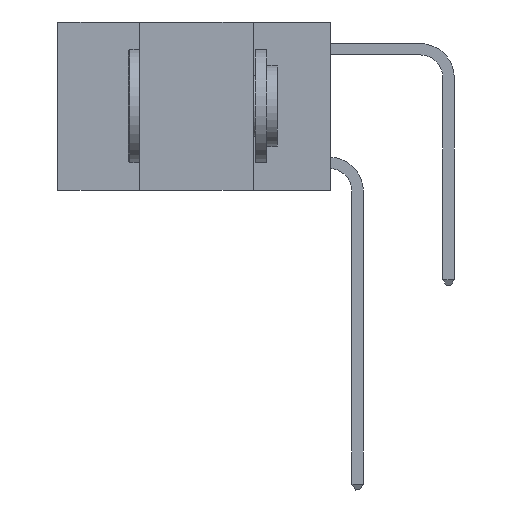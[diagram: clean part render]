
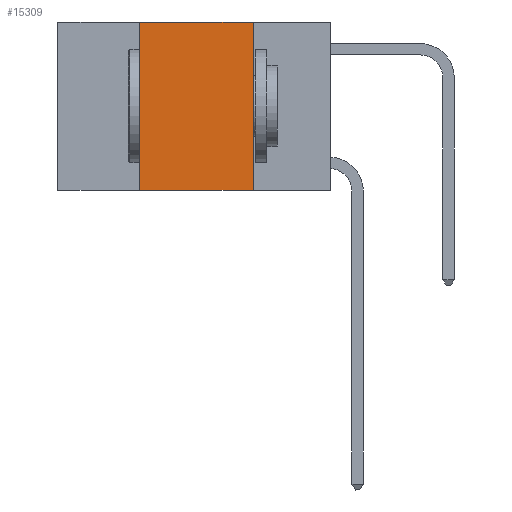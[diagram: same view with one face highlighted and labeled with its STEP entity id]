
A CAD part, left-side view. The second image highlights one B-rep face of the part: STEP entity #15309.
In plain terms, the highlighted planar face has unit normal (-1, 0, 0).
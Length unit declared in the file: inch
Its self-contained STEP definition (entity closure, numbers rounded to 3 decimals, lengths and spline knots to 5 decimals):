
#943 = LINE ( 'NONE', #4119, #15385 ) ;
#1379 = EDGE_CURVE ( 'NONE', #6862, #9455, #2461, .T. ) ;
#2232 = CARTESIAN_POINT ( 'NONE',  ( 0., 0.42, 0. ) ) ;
#2461 = LINE ( 'NONE', #2232, #5906 ) ;
#3121 = LINE ( 'NONE', #6906, #5429 ) ;
#4119 = CARTESIAN_POINT ( 'NONE',  ( 0., 0.17, 0. ) ) ;
#5046 = ORIENTED_EDGE ( 'NONE', *, *, #7975, .F. ) ;
#5420 = EDGE_CURVE ( 'NONE', #6862, #9086, #3121, .T. ) ;
#5429 = VECTOR ( 'NONE', #12276, 39.37008 ) ;
#5552 = DIRECTION ( 'NONE',  ( 0., 0., 1. ) ) ;
#5906 = VECTOR ( 'NONE', #5552, 39.37008 ) ;
#6086 = CARTESIAN_POINT ( 'NONE',  ( 0., 0.6, 0. ) ) ;
#6357 = DIRECTION ( 'NONE',  ( 0., 0., -1. ) ) ;
#6862 = VERTEX_POINT ( 'NONE', #23039 ) ;
#6906 = CARTESIAN_POINT ( 'NONE',  ( 0., 0.6, -0.37 ) ) ;
#6937 = DIRECTION ( 'NONE',  ( 0., 0., -1. ) ) ;
#7040 = EDGE_CURVE ( 'NONE', #17210, #9086, #943, .T. ) ;
#7322 = ORIENTED_EDGE ( 'NONE', *, *, #5420, .T. ) ;
#7428 = ORIENTED_EDGE ( 'NONE', *, *, #1379, .F. ) ;
#7971 = DIRECTION ( 'NONE',  ( 0., -1., 0. ) ) ;
#7975 = EDGE_CURVE ( 'NONE', #9455, #17210, #20556, .T. ) ;
#9086 = VERTEX_POINT ( 'NONE', #12196 ) ;
#9203 = AXIS2_PLACEMENT_3D ( 'NONE', #11604, #15391, #6937 ) ;
#9455 = VERTEX_POINT ( 'NONE', #22393 ) ;
#9873 = FACE_OUTER_BOUND ( 'NONE', #10589, .T. ) ;
#10589 = EDGE_LOOP ( 'NONE', ( #14889, #5046, #7428, #7322 ) ) ;
#11604 = CARTESIAN_POINT ( 'NONE',  ( 0., 0.6, 0. ) ) ;
#11678 = VECTOR ( 'NONE', #7971, 39.37008 ) ;
#12196 = CARTESIAN_POINT ( 'NONE',  ( 0., 0.17, -0.37 ) ) ;
#12276 = DIRECTION ( 'NONE',  ( 0., -1., 0. ) ) ;
#13310 = CARTESIAN_POINT ( 'NONE',  ( 0., 0.17, 0. ) ) ;
#14889 = ORIENTED_EDGE ( 'NONE', *, *, #7040, .F. ) ;
#15309 = ADVANCED_FACE ( 'NONE', ( #9873 ), #17134, .F. ) ;
#15385 = VECTOR ( 'NONE', #6357, 39.37008 ) ;
#15391 = DIRECTION ( 'NONE',  ( 1., 0., 0. ) ) ;
#17134 = PLANE ( 'NONE',  #9203 ) ;
#17210 = VERTEX_POINT ( 'NONE', #13310 ) ;
#20556 = LINE ( 'NONE', #6086, #11678 ) ;
#22393 = CARTESIAN_POINT ( 'NONE',  ( 0., 0.42, 0. ) ) ;
#23039 = CARTESIAN_POINT ( 'NONE',  ( 0., 0.42, -0.37 ) ) ;
